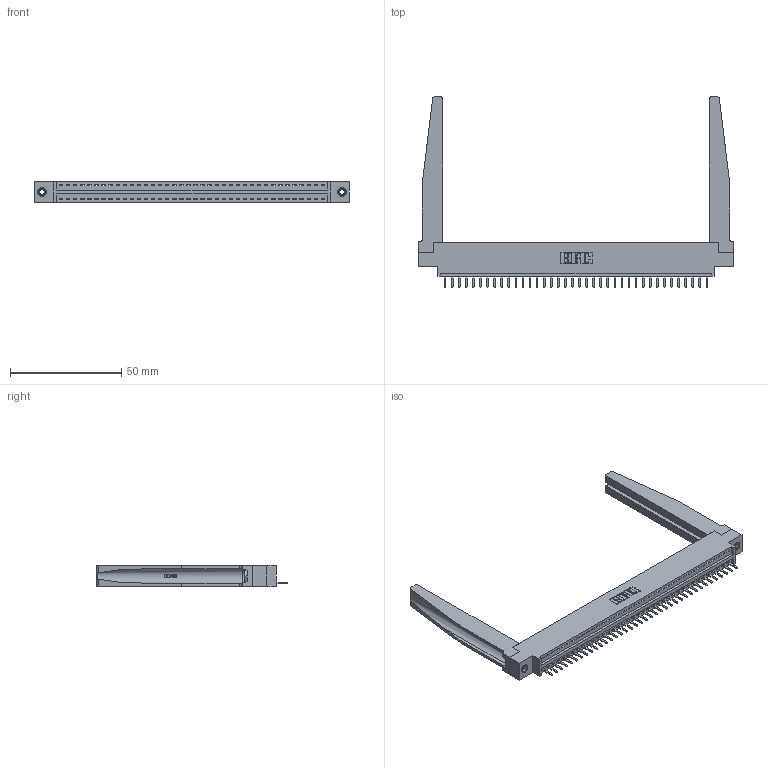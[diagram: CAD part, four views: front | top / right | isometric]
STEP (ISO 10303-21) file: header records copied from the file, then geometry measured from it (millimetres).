
FILE_DESCRIPTION (( 'STEP AP203' ), '1' );
FILE_NAME ('396-038-520-678.STEP', '2019-10-27T18:12:00', ( '' ), ( '' ), 'SwSTEP 2.0', 'SolidWorks 2016', '' );
FILE_SCHEMA (( 'CONFIG_CONTROL_DESIGN' ));
Length unit declared in the file: inch
Products named in the file (5): 346-220-078_345-220-078; 345-250-001_345-250-001-102; 345-292-001_345-293-120; 396-038-520-678; 346 Part_0.170 Offset - 0.156 Dia-TH
Assembly tree (43 placements, depth 2):
  396-038-520-678
    346 Part_0.170 Offset - 0.156 Dia-TH
    345-292-001_345-293-120  x38
    346-220-078_345-220-078  x2
    345-250-001_345-250-001-102  x2
Bounding box: 141.22 x 85.29 x 9.4 mm (x, y, z)
Volume: 20135.6 mm3; surface area: 22824.1 mm2
Topology: 43 solids, 43 shells, 2716 faces, 7941 edges, 5182 vertices
Faces by surface type: plane 1818, cylinder 846, bspline 36, cone 12, torus 4
Entity records: 29116 total; most frequent: CARTESIAN_POINT 5917, ORIENTED_EDGE 4766, DIRECTION 4197, EDGE_CURVE 2383, VECTOR 2001, LINE 2001, VERTEX_POINT 1580, AXIS2_PLACEMENT_3D 1098
